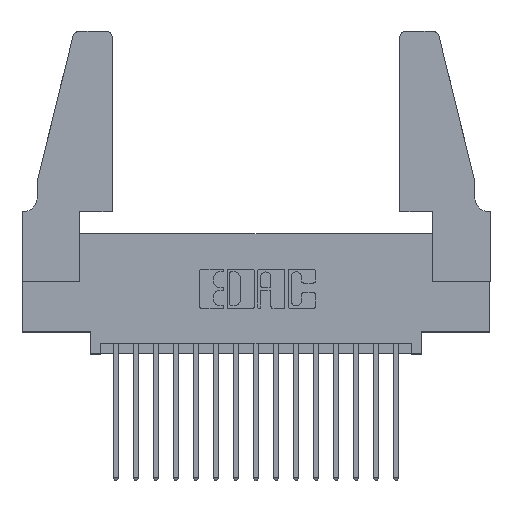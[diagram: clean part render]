
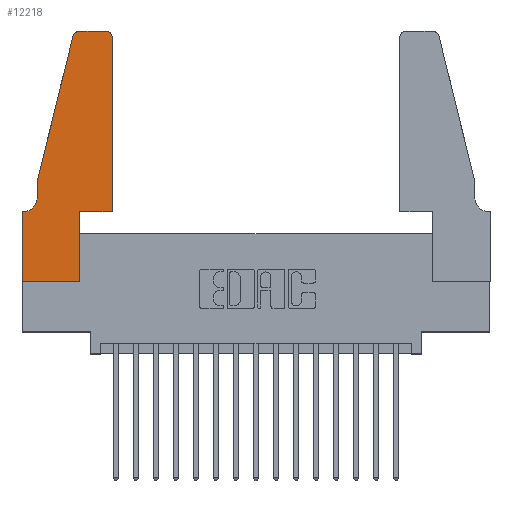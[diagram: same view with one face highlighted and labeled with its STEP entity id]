
A CAD part, top view. The second image highlights one B-rep face of the part: STEP entity #12218.
In plain terms, the highlighted planar face has unit normal (0, 0, 1).
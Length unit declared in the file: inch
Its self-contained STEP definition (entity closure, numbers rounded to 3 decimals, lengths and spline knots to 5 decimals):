
#55 = EDGE_CURVE ( 'NONE', #6652, #1201, #1876, .T. ) ;
#66 = VERTEX_POINT ( 'NONE', #4618 ) ;
#78 = DIRECTION ( 'NONE',  ( 0., 1., 0. ) ) ;
#332 = VECTOR ( 'NONE', #10855, 39.37008 ) ;
#348 = EDGE_CURVE ( 'NONE', #16226, #2721, #4245, .T. ) ;
#784 = CARTESIAN_POINT ( 'NONE',  ( 0.2865, 0., 0.37 ) ) ;
#964 = DIRECTION ( 'NONE',  ( -1., 0., 0. ) ) ;
#1131 = VECTOR ( 'NONE', #13488, 39.37008 ) ;
#1201 = VERTEX_POINT ( 'NONE', #1666 ) ;
#1435 = CARTESIAN_POINT ( 'NONE',  ( 0.4505, 0.35, 0.37 ) ) ;
#1619 = AXIS2_PLACEMENT_3D ( 'NONE', #9102, #11946, #964 ) ;
#1666 = CARTESIAN_POINT ( 'NONE',  ( 0.0755, 0.42, 0.37 ) ) ;
#1695 = EDGE_CURVE ( 'NONE', #8834, #12145, #5260, .T. ) ;
#1817 = CARTESIAN_POINT ( 'NONE',  ( 0.4505, 0.35, 0.37 ) ) ;
#1876 = LINE ( 'NONE', #7378, #16051 ) ;
#2164 = ORIENTED_EDGE ( 'NONE', *, *, #13795, .T. ) ;
#2201 = CARTESIAN_POINT ( 'NONE',  ( 0., 0.35, 0.37 ) ) ;
#2525 = LINE ( 'NONE', #1435, #6655 ) ;
#2574 = CARTESIAN_POINT ( 'NONE',  ( 0.0055, 0.35, 0.37 ) ) ;
#2721 = VERTEX_POINT ( 'NONE', #784 ) ;
#2955 = EDGE_CURVE ( 'NONE', #5089, #16226, #3251, .T. ) ;
#3102 = ORIENTED_EDGE ( 'NONE', *, *, #4324, .T. ) ;
#3165 = VERTEX_POINT ( 'NONE', #16767 ) ;
#3251 = LINE ( 'NONE', #13368, #1131 ) ;
#3335 = ORIENTED_EDGE ( 'NONE', *, *, #5167, .T. ) ;
#3368 = ORIENTED_EDGE ( 'NONE', *, *, #9596, .T. ) ;
#3455 = CARTESIAN_POINT ( 'NONE',  ( 0.25487, 1.22718, 0.37 ) ) ;
#3547 = CARTESIAN_POINT ( 'NONE',  ( 0.284, 1.22, 0.37 ) ) ;
#3597 = CARTESIAN_POINT ( 'NONE',  ( 0.2865, 0.35, 0.37 ) ) ;
#4245 = LINE ( 'NONE', #16460, #9606 ) ;
#4283 = CARTESIAN_POINT ( 'NONE',  ( 0.4205, 1.25, 0.37 ) ) ;
#4324 = EDGE_CURVE ( 'NONE', #3165, #6711, #11362, .T. ) ;
#4553 = DIRECTION ( 'NONE',  ( -1., 0., 0. ) ) ;
#4618 = CARTESIAN_POINT ( 'NONE',  ( 0.4505, 0.35, 0.37 ) ) ;
#4931 = DIRECTION ( 'NONE',  ( 1., 0., 0. ) ) ;
#4974 = ORIENTED_EDGE ( 'NONE', *, *, #2955, .T. ) ;
#4989 = CARTESIAN_POINT ( 'NONE',  ( 0., 0.35, 0.37 ) ) ;
#5043 = EDGE_CURVE ( 'NONE', #6417, #5089, #11136, .T. ) ;
#5053 = CARTESIAN_POINT ( 'NONE',  ( 0.0755, 0.35, 0.37 ) ) ;
#5089 = VERTEX_POINT ( 'NONE', #4989 ) ;
#5167 = EDGE_CURVE ( 'NONE', #1201, #6417, #12622, .T. ) ;
#5260 = CIRCLE ( 'NONE', #11443, 0.03 ) ;
#5713 = ORIENTED_EDGE ( 'NONE', *, *, #15730, .T. ) ;
#6382 = CARTESIAN_POINT ( 'NONE',  ( 0.0755, 0.5, 0.37 ) ) ;
#6417 = VERTEX_POINT ( 'NONE', #2574 ) ;
#6442 = EDGE_CURVE ( 'NONE', #2721, #9119, #11210, .T. ) ;
#6652 = VERTEX_POINT ( 'NONE', #15335 ) ;
#6655 = VECTOR ( 'NONE', #78, 39.37008 ) ;
#6696 = VECTOR ( 'NONE', #7752, 39.37008 ) ;
#6711 = VERTEX_POINT ( 'NONE', #4283 ) ;
#6909 = VECTOR ( 'NONE', #13312, 39.37008 ) ;
#7378 = CARTESIAN_POINT ( 'NONE',  ( 0.0755, 0.5, 0.37 ) ) ;
#7450 = DIRECTION ( 'NONE',  ( 1., 0., 0. ) ) ;
#7535 = DIRECTION ( 'NONE',  ( 1., 0., 0. ) ) ;
#7724 = DIRECTION ( 'NONE',  ( 1., 0., 0. ) ) ;
#7752 = DIRECTION ( 'NONE',  ( -0.239, -0.971, 0. ) ) ;
#8803 = AXIS2_PLACEMENT_3D ( 'NONE', #2201, #13139, #4931 ) ;
#8834 = VERTEX_POINT ( 'NONE', #11382 ) ;
#9102 = CARTESIAN_POINT ( 'NONE',  ( 0.0055, 0.42, 0.37 ) ) ;
#9108 = PLANE ( 'NONE',  #8803 ) ;
#9119 = VERTEX_POINT ( 'NONE', #3597 ) ;
#9234 = VECTOR ( 'NONE', #7535, 39.37008 ) ;
#9462 = LINE ( 'NONE', #1817, #9234 ) ;
#9596 = EDGE_CURVE ( 'NONE', #12145, #6652, #15204, .T. ) ;
#9606 = VECTOR ( 'NONE', #13543, 39.37008 ) ;
#10434 = EDGE_LOOP ( 'NONE', ( #2164, #13736, #3368, #16414, #3335, #12545, #4974, #12978, #15081, #5713, #15867, #3102 ) ) ;
#10855 = DIRECTION ( 'NONE',  ( 0., 1., 0. ) ) ;
#11136 = LINE ( 'NONE', #5053, #6909 ) ;
#11210 = LINE ( 'NONE', #16187, #332 ) ;
#11362 = CIRCLE ( 'NONE', #14915, 0.03 ) ;
#11382 = CARTESIAN_POINT ( 'NONE',  ( 0.284, 1.25, 0.37 ) ) ;
#11422 = DIRECTION ( 'NONE',  ( 0., -1., 0. ) ) ;
#11443 = AXIS2_PLACEMENT_3D ( 'NONE', #3547, #17390, #7724 ) ;
#11467 = CARTESIAN_POINT ( 'NONE',  ( 0.2605, 1.25, 0.37 ) ) ;
#11946 = DIRECTION ( 'NONE',  ( 0., 0., -1. ) ) ;
#12106 = FACE_OUTER_BOUND ( 'NONE', #10434, .T. ) ;
#12145 = VERTEX_POINT ( 'NONE', #3455 ) ;
#12218 = ADVANCED_FACE ( 'NONE', ( #12106 ), #9108, .T. ) ;
#12545 = ORIENTED_EDGE ( 'NONE', *, *, #5043, .T. ) ;
#12622 = CIRCLE ( 'NONE', #1619, 0.07 ) ;
#12671 = DIRECTION ( 'NONE',  ( 0., 0., 1. ) ) ;
#12978 = ORIENTED_EDGE ( 'NONE', *, *, #348, .T. ) ;
#13139 = DIRECTION ( 'NONE',  ( 0., 0., 1. ) ) ;
#13312 = DIRECTION ( 'NONE',  ( -1., 0., 0. ) ) ;
#13368 = CARTESIAN_POINT ( 'NONE',  ( 0., 0., 0.37 ) ) ;
#13488 = DIRECTION ( 'NONE',  ( 0., -1., 0. ) ) ;
#13543 = DIRECTION ( 'NONE',  ( 1., 0., 0. ) ) ;
#13736 = ORIENTED_EDGE ( 'NONE', *, *, #1695, .T. ) ;
#13795 = EDGE_CURVE ( 'NONE', #6711, #8834, #17418, .T. ) ;
#14915 = AXIS2_PLACEMENT_3D ( 'NONE', #16786, #12671, #7450 ) ;
#15081 = ORIENTED_EDGE ( 'NONE', *, *, #6442, .T. ) ;
#15204 = LINE ( 'NONE', #6382, #6696 ) ;
#15335 = CARTESIAN_POINT ( 'NONE',  ( 0.0755, 0.5, 0.37 ) ) ;
#15730 = EDGE_CURVE ( 'NONE', #9119, #66, #9462, .T. ) ;
#15867 = ORIENTED_EDGE ( 'NONE', *, *, #17053, .T. ) ;
#15916 = VECTOR ( 'NONE', #4553, 39.37008 ) ;
#16051 = VECTOR ( 'NONE', #11422, 39.37008 ) ;
#16187 = CARTESIAN_POINT ( 'NONE',  ( 0.2865, 0.35, 0.37 ) ) ;
#16226 = VERTEX_POINT ( 'NONE', #17114 ) ;
#16414 = ORIENTED_EDGE ( 'NONE', *, *, #55, .T. ) ;
#16460 = CARTESIAN_POINT ( 'NONE',  ( 0., 0., 0.37 ) ) ;
#16767 = CARTESIAN_POINT ( 'NONE',  ( 0.4505, 1.22, 0.37 ) ) ;
#16786 = CARTESIAN_POINT ( 'NONE',  ( 0.4205, 1.22, 0.37 ) ) ;
#17053 = EDGE_CURVE ( 'NONE', #66, #3165, #2525, .T. ) ;
#17114 = CARTESIAN_POINT ( 'NONE',  ( 0., 0., 0.37 ) ) ;
#17390 = DIRECTION ( 'NONE',  ( 0., 0., 1. ) ) ;
#17418 = LINE ( 'NONE', #11467, #15916 ) ;
